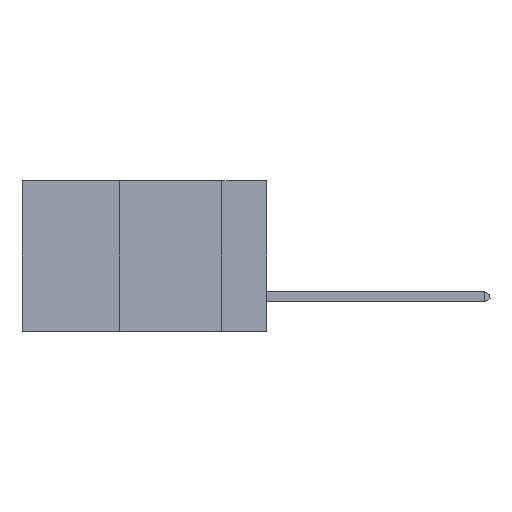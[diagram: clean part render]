
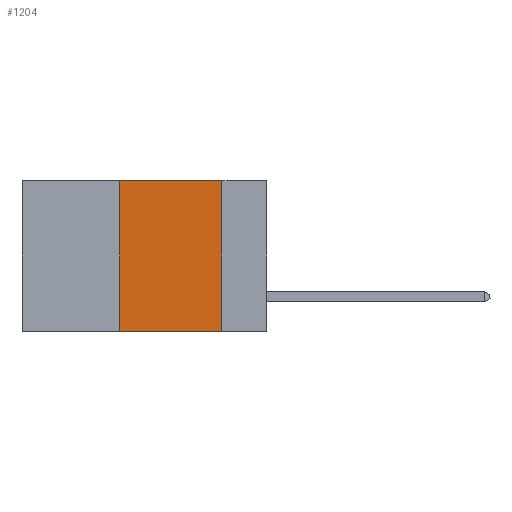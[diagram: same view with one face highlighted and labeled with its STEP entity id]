
A CAD part, left-side view. The second image highlights one B-rep face of the part: STEP entity #1204.
In plain terms, the highlighted planar face has unit normal (-1, 0, 0).
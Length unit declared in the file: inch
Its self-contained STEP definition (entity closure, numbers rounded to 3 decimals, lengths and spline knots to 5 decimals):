
#208 = LINE ( 'NONE', #13304, #8575 ) ;
#848 = DIRECTION ( 'NONE',  ( 0., -1., 0. ) ) ;
#928 = VERTEX_POINT ( 'NONE', #13053 ) ;
#1204 = ADVANCED_FACE ( 'NONE', ( #14101 ), #18775, .F. ) ;
#1284 = DIRECTION ( 'NONE',  ( 0., -1., 0. ) ) ;
#1711 = LINE ( 'NONE', #18368, #2814 ) ;
#2595 = DIRECTION ( 'NONE',  ( 1., 0., 0. ) ) ;
#2693 = VECTOR ( 'NONE', #17598, 39.37008 ) ;
#2814 = VECTOR ( 'NONE', #1284, 39.37008 ) ;
#4368 = DIRECTION ( 'NONE',  ( 0., 0., -1. ) ) ;
#4808 = VECTOR ( 'NONE', #848, 39.37008 ) ;
#6534 = EDGE_CURVE ( 'NONE', #928, #10688, #1711, .T. ) ;
#6896 = CARTESIAN_POINT ( 'NONE',  ( 0., 0.11, -0.37 ) ) ;
#8575 = VECTOR ( 'NONE', #21632, 39.37008 ) ;
#10248 = CARTESIAN_POINT ( 'NONE',  ( 0., 0.6, 0. ) ) ;
#10546 = EDGE_CURVE ( 'NONE', #10688, #19904, #208, .T. ) ;
#10688 = VERTEX_POINT ( 'NONE', #18734 ) ;
#11277 = AXIS2_PLACEMENT_3D ( 'NONE', #10248, #2595, #4368 ) ;
#12065 = ORIENTED_EDGE ( 'NONE', *, *, #20379, .T. ) ;
#13053 = CARTESIAN_POINT ( 'NONE',  ( 0., 0.36, 0. ) ) ;
#13304 = CARTESIAN_POINT ( 'NONE',  ( 0., 0.11, 0. ) ) ;
#14101 = FACE_OUTER_BOUND ( 'NONE', #17498, .T. ) ;
#14258 = CARTESIAN_POINT ( 'NONE',  ( 0., 0.36, 0. ) ) ;
#14495 = ORIENTED_EDGE ( 'NONE', *, *, #10546, .F. ) ;
#14611 = CARTESIAN_POINT ( 'NONE',  ( 0., 0.36, -0.37 ) ) ;
#17268 = LINE ( 'NONE', #14258, #2693 ) ;
#17498 = EDGE_LOOP ( 'NONE', ( #14495, #19922, #17917, #12065 ) ) ;
#17598 = DIRECTION ( 'NONE',  ( 0., 0., 1. ) ) ;
#17917 = ORIENTED_EDGE ( 'NONE', *, *, #22043, .F. ) ;
#18368 = CARTESIAN_POINT ( 'NONE',  ( 0., 0.6, 0. ) ) ;
#18385 = CARTESIAN_POINT ( 'NONE',  ( 0., 0.6, -0.37 ) ) ;
#18696 = LINE ( 'NONE', #18385, #4808 ) ;
#18734 = CARTESIAN_POINT ( 'NONE',  ( 0., 0.11, 0. ) ) ;
#18775 = PLANE ( 'NONE',  #11277 ) ;
#19657 = VERTEX_POINT ( 'NONE', #14611 ) ;
#19904 = VERTEX_POINT ( 'NONE', #6896 ) ;
#19922 = ORIENTED_EDGE ( 'NONE', *, *, #6534, .F. ) ;
#20379 = EDGE_CURVE ( 'NONE', #19657, #19904, #18696, .T. ) ;
#21632 = DIRECTION ( 'NONE',  ( 0., 0., -1. ) ) ;
#22043 = EDGE_CURVE ( 'NONE', #19657, #928, #17268, .T. ) ;
